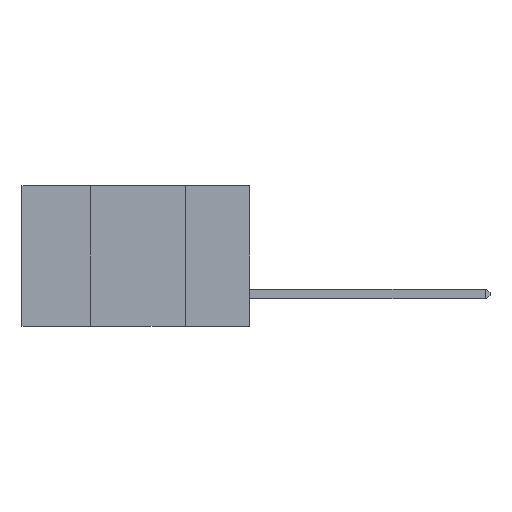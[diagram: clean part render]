
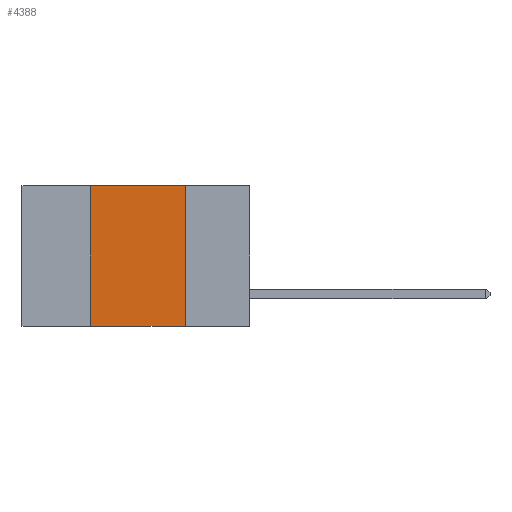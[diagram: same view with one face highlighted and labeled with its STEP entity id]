
A CAD part, left-side view. The second image highlights one B-rep face of the part: STEP entity #4388.
In plain terms, the highlighted planar face has unit normal (-1, 0, 0).
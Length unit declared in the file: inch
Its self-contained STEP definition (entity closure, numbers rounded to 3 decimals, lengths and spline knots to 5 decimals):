
#81 = CARTESIAN_POINT ( 'NONE',  ( 0., 0.17, 0. ) ) ;
#293 = VERTEX_POINT ( 'NONE', #4548 ) ;
#410 = VERTEX_POINT ( 'NONE', #4258 ) ;
#553 = ORIENTED_EDGE ( 'NONE', *, *, #8302, .F. ) ;
#580 = VECTOR ( 'NONE', #9412, 39.37008 ) ;
#670 = EDGE_CURVE ( 'NONE', #4664, #3264, #8627, .T. ) ;
#877 = ORIENTED_EDGE ( 'NONE', *, *, #8303, .F. ) ;
#879 = LINE ( 'NONE', #8813, #580 ) ;
#1903 = EDGE_LOOP ( 'NONE', ( #3564, #553, #877, #5468 ) ) ;
#2363 = FACE_OUTER_BOUND ( 'NONE', #1903, .T. ) ;
#2829 = DIRECTION ( 'NONE',  ( 0., 0., -1. ) ) ;
#2885 = CARTESIAN_POINT ( 'NONE',  ( 0., 0.6, -0.37 ) ) ;
#2891 = DIRECTION ( 'NONE',  ( 0., -1., 0. ) ) ;
#3264 = VERTEX_POINT ( 'NONE', #3722 ) ;
#3564 = ORIENTED_EDGE ( 'NONE', *, *, #7879, .F. ) ;
#3722 = CARTESIAN_POINT ( 'NONE',  ( 0., 0.17, -0.37 ) ) ;
#4258 = CARTESIAN_POINT ( 'NONE',  ( 0., 0.17, 0. ) ) ;
#4388 = ADVANCED_FACE ( 'NONE', ( #2363 ), #7446, .F. ) ;
#4548 = CARTESIAN_POINT ( 'NONE',  ( 0., 0.42, 0. ) ) ;
#4664 = VERTEX_POINT ( 'NONE', #5948 ) ;
#4990 = VECTOR ( 'NONE', #2829, 39.37008 ) ;
#5107 = LINE ( 'NONE', #6230, #6494 ) ;
#5468 = ORIENTED_EDGE ( 'NONE', *, *, #670, .T. ) ;
#5948 = CARTESIAN_POINT ( 'NONE',  ( 0., 0.42, -0.37 ) ) ;
#6230 = CARTESIAN_POINT ( 'NONE',  ( 0., 0.42, 0. ) ) ;
#6494 = VECTOR ( 'NONE', #6898, 39.37008 ) ;
#6898 = DIRECTION ( 'NONE',  ( 0., 0., 1. ) ) ;
#7213 = LINE ( 'NONE', #81, #4990 ) ;
#7446 = PLANE ( 'NONE',  #8218 ) ;
#7733 = DIRECTION ( 'NONE',  ( 1., 0., 0. ) ) ;
#7778 = DIRECTION ( 'NONE',  ( 0., 0., -1. ) ) ;
#7879 = EDGE_CURVE ( 'NONE', #410, #3264, #7213, .T. ) ;
#8218 = AXIS2_PLACEMENT_3D ( 'NONE', #8341, #7733, #7778 ) ;
#8302 = EDGE_CURVE ( 'NONE', #293, #410, #879, .T. ) ;
#8303 = EDGE_CURVE ( 'NONE', #4664, #293, #5107, .T. ) ;
#8341 = CARTESIAN_POINT ( 'NONE',  ( 0., 0.6, 0. ) ) ;
#8437 = VECTOR ( 'NONE', #2891, 39.37008 ) ;
#8627 = LINE ( 'NONE', #2885, #8437 ) ;
#8813 = CARTESIAN_POINT ( 'NONE',  ( 0., 0.6, 0. ) ) ;
#9412 = DIRECTION ( 'NONE',  ( 0., -1., 0. ) ) ;
